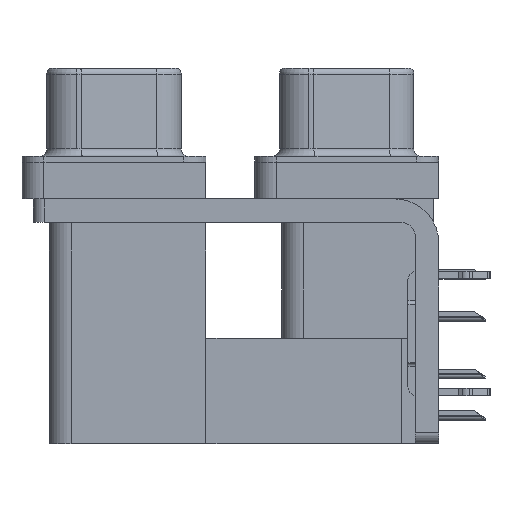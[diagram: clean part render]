
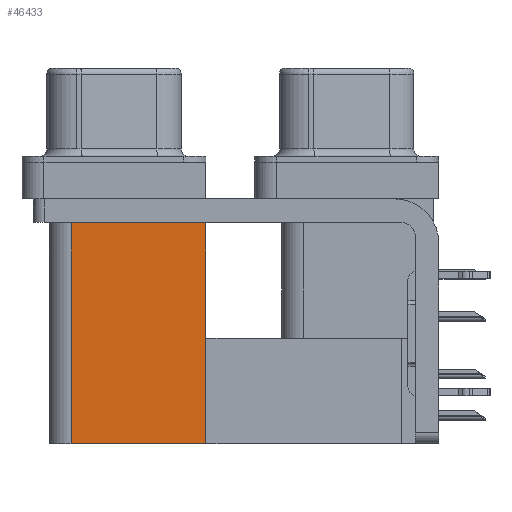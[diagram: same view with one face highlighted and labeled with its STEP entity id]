
A CAD part, left-side view. The second image highlights one B-rep face of the part: STEP entity #46433.
In plain terms, the highlighted planar face has unit normal (-1, 0, 0).
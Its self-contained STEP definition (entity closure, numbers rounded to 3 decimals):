
#3716 = EDGE_LOOP ( 'NONE', ( #34758, #23188, #34291, #10425 ) ) ;
#4069 = EDGE_CURVE ( 'NONE', #46993, #26172, #32971, .T. ) ;
#5832 = CARTESIAN_POINT ( 'NONE',  ( 3.79, 9.6, -2.5 ) ) ;
#8330 = VECTOR ( 'NONE', #48968, 1000. ) ;
#8761 = EDGE_CURVE ( 'NONE', #12758, #26172, #25473, .T. ) ;
#9135 = EDGE_CURVE ( 'NONE', #42328, #46993, #48555, .T. ) ;
#9196 = CARTESIAN_POINT ( 'NONE',  ( 3.79, 18.8, -19.2 ) ) ;
#10069 = CARTESIAN_POINT ( 'NONE',  ( 3.79, 9.6, -19.2 ) ) ;
#10425 = ORIENTED_EDGE ( 'NONE', *, *, #9135, .T. ) ;
#12758 = VERTEX_POINT ( 'NONE', #22865 ) ;
#13441 = DIRECTION ( 'NONE',  ( 0., 1., 0. ) ) ;
#13899 = CARTESIAN_POINT ( 'NONE',  ( 3.79, 18.8, -2.5 ) ) ;
#15063 = DIRECTION ( 'NONE',  ( 0., 0., -1. ) ) ;
#20932 = CARTESIAN_POINT ( 'NONE',  ( 3.79, 9.6, -19.2 ) ) ;
#22329 = CARTESIAN_POINT ( 'NONE',  ( 3.79, 9.6, -19.2 ) ) ;
#22838 = FACE_OUTER_BOUND ( 'NONE', #3716, .T. ) ;
#22865 = CARTESIAN_POINT ( 'NONE',  ( 3.79, 18.8, -19.2 ) ) ;
#23188 = ORIENTED_EDGE ( 'NONE', *, *, #8761, .F. ) ;
#23348 = CARTESIAN_POINT ( 'NONE',  ( 3.79, 9.6, -19.2 ) ) ;
#25473 = LINE ( 'NONE', #9196, #42010 ) ;
#25753 = EDGE_CURVE ( 'NONE', #42328, #12758, #26375, .T. ) ;
#26172 = VERTEX_POINT ( 'NONE', #13899 ) ;
#26375 = LINE ( 'NONE', #10069, #32606 ) ;
#26526 = VECTOR ( 'NONE', #28187, 1000. ) ;
#28187 = DIRECTION ( 'NONE',  ( 0., 0., 1. ) ) ;
#32606 = VECTOR ( 'NONE', #13441, 1000. ) ;
#32971 = LINE ( 'NONE', #5832, #8330 ) ;
#34291 = ORIENTED_EDGE ( 'NONE', *, *, #25753, .F. ) ;
#34758 = ORIENTED_EDGE ( 'NONE', *, *, #4069, .T. ) ;
#35290 = AXIS2_PLACEMENT_3D ( 'NONE', #22329, #38571, #15063 ) ;
#38051 = PLANE ( 'NONE',  #35290 ) ;
#38571 = DIRECTION ( 'NONE',  ( 1., 0., 0. ) ) ;
#42010 = VECTOR ( 'NONE', #44820, 1000. ) ;
#42328 = VERTEX_POINT ( 'NONE', #23348 ) ;
#44820 = DIRECTION ( 'NONE',  ( 0., 0., 1. ) ) ;
#46433 = ADVANCED_FACE ( 'NONE', ( #22838 ), #38051, .F. ) ;
#46993 = VERTEX_POINT ( 'NONE', #49946 ) ;
#48555 = LINE ( 'NONE', #20932, #26526 ) ;
#48968 = DIRECTION ( 'NONE',  ( 0., 1., 0. ) ) ;
#49946 = CARTESIAN_POINT ( 'NONE',  ( 3.79, 9.6, -2.5 ) ) ;
